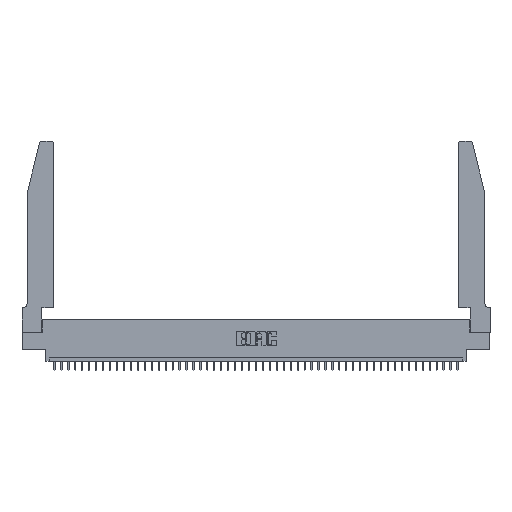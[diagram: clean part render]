
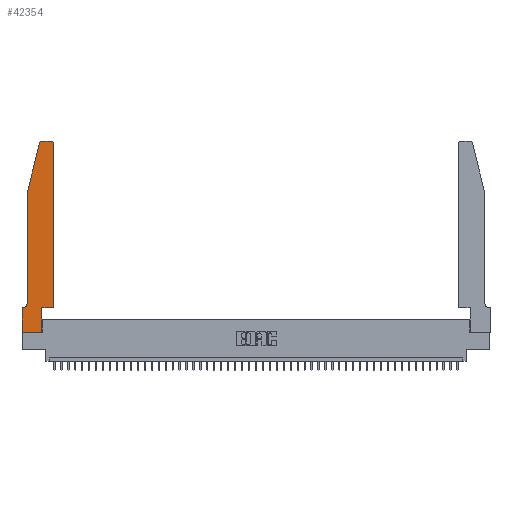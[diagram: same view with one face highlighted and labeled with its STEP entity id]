
A CAD part, top view. The second image highlights one B-rep face of the part: STEP entity #42354.
In plain terms, the highlighted planar face has unit normal (0, 0, 1).
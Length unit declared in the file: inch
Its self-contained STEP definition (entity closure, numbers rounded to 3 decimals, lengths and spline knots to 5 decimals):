
#681 = ORIENTED_EDGE ( 'NONE', *, *, #24891, .T. ) ;
#695 = CARTESIAN_POINT ( 'NONE',  ( 0.2865, 0., 0.37 ) ) ;
#1865 = CARTESIAN_POINT ( 'NONE',  ( 0.2865, 0.35, 0.37 ) ) ;
#1899 = EDGE_CURVE ( 'NONE', #6801, #45383, #42793, .T. ) ;
#1970 = DIRECTION ( 'NONE',  ( 0., 1., 0. ) ) ;
#2042 = EDGE_CURVE ( 'NONE', #19878, #34717, #4659, .T. ) ;
#2085 = VECTOR ( 'NONE', #27635, 39.37008 ) ;
#2311 = EDGE_CURVE ( 'NONE', #34717, #32950, #13893, .T. ) ;
#2432 = CARTESIAN_POINT ( 'NONE',  ( 0.2865, 0.35, 0.37 ) ) ;
#2750 = EDGE_CURVE ( 'NONE', #32636, #19404, #9795, .T. ) ;
#2810 = ORIENTED_EDGE ( 'NONE', *, *, #10127, .T. ) ;
#3376 = ORIENTED_EDGE ( 'NONE', *, *, #11991, .T. ) ;
#3710 = CARTESIAN_POINT ( 'NONE',  ( 0.2605, 2.75, 0.37 ) ) ;
#4659 = LINE ( 'NONE', #19162, #28533 ) ;
#5027 = AXIS2_PLACEMENT_3D ( 'NONE', #43188, #36262, #32211 ) ;
#6279 = DIRECTION ( 'NONE',  ( 0., 0., 1. ) ) ;
#6488 = DIRECTION ( 'NONE',  ( 1., 0., 0. ) ) ;
#6801 = VERTEX_POINT ( 'NONE', #29348 ) ;
#7514 = CARTESIAN_POINT ( 'NONE',  ( 0.4505, 2.72, 0.37 ) ) ;
#7860 = LINE ( 'NONE', #22376, #17465 ) ;
#8161 = DIRECTION ( 'NONE',  ( 1., 0., 0. ) ) ;
#8250 = ORIENTED_EDGE ( 'NONE', *, *, #2042, .T. ) ;
#8858 = CIRCLE ( 'NONE', #11123, 0.07 ) ;
#8876 = LINE ( 'NONE', #44636, #16606 ) ;
#9313 = LINE ( 'NONE', #38373, #2085 ) ;
#9795 = LINE ( 'NONE', #31712, #18900 ) ;
#9813 = LINE ( 'NONE', #2432, #31734 ) ;
#9866 = VECTOR ( 'NONE', #10618, 39.37008 ) ;
#10078 = CARTESIAN_POINT ( 'NONE',  ( 0., 0., 0.37 ) ) ;
#10095 = ORIENTED_EDGE ( 'NONE', *, *, #46100, .T. ) ;
#10127 = EDGE_CURVE ( 'NONE', #16687, #29132, #9813, .T. ) ;
#10618 = DIRECTION ( 'NONE',  ( -1., 0., 0. ) ) ;
#11123 = AXIS2_PLACEMENT_3D ( 'NONE', #24997, #31701, #39310 ) ;
#11627 = ORIENTED_EDGE ( 'NONE', *, *, #2750, .T. ) ;
#11991 = EDGE_CURVE ( 'NONE', #43808, #40932, #9313, .T. ) ;
#13331 = CARTESIAN_POINT ( 'NONE',  ( 0.0055, 0.35, 0.37 ) ) ;
#13660 = CARTESIAN_POINT ( 'NONE',  ( 0., 0., 0.37 ) ) ;
#13893 = LINE ( 'NONE', #13660, #29370 ) ;
#14557 = EDGE_CURVE ( 'NONE', #29132, #43808, #7860, .T. ) ;
#16606 = VECTOR ( 'NONE', #8161, 39.37008 ) ;
#16687 = VERTEX_POINT ( 'NONE', #695 ) ;
#16917 = ORIENTED_EDGE ( 'NONE', *, *, #1899, .T. ) ;
#17465 = VECTOR ( 'NONE', #6488, 39.37008 ) ;
#17757 = CARTESIAN_POINT ( 'NONE',  ( 0., 0.35, 0.37 ) ) ;
#18342 = CARTESIAN_POINT ( 'NONE',  ( 0., 0.35, 0.37 ) ) ;
#18900 = VECTOR ( 'NONE', #20962, 39.37008 ) ;
#19162 = CARTESIAN_POINT ( 'NONE',  ( 0.0755, 0.35, 0.37 ) ) ;
#19404 = VERTEX_POINT ( 'NONE', #20272 ) ;
#19878 = VERTEX_POINT ( 'NONE', #13331 ) ;
#20091 = CARTESIAN_POINT ( 'NONE',  ( 0.4205, 2.72, 0.37 ) ) ;
#20272 = CARTESIAN_POINT ( 'NONE',  ( 0.0755, 2., 0.37 ) ) ;
#20962 = DIRECTION ( 'NONE',  ( -0.239, -0.971, 0. ) ) ;
#21326 = FACE_OUTER_BOUND ( 'NONE', #31889, .T. ) ;
#21738 = ORIENTED_EDGE ( 'NONE', *, *, #45630, .T. ) ;
#22376 = CARTESIAN_POINT ( 'NONE',  ( 0.4505, 0.35, 0.37 ) ) ;
#23330 = CARTESIAN_POINT ( 'NONE',  ( 0.0755, 0.42, 0.37 ) ) ;
#23818 = VECTOR ( 'NONE', #33540, 39.37008 ) ;
#24444 = VERTEX_POINT ( 'NONE', #23330 ) ;
#24891 = EDGE_CURVE ( 'NONE', #40932, #6801, #43857, .T. ) ;
#24997 = CARTESIAN_POINT ( 'NONE',  ( 0.0055, 0.42, 0.37 ) ) ;
#27635 = DIRECTION ( 'NONE',  ( 0., 1., 0. ) ) ;
#28533 = VECTOR ( 'NONE', #36586, 39.37008 ) ;
#28964 = DIRECTION ( 'NONE',  ( 1., 0., 0. ) ) ;
#29119 = AXIS2_PLACEMENT_3D ( 'NONE', #17757, #32294, #28964 ) ;
#29132 = VERTEX_POINT ( 'NONE', #1865 ) ;
#29185 = CARTESIAN_POINT ( 'NONE',  ( 0.25487, 2.72718, 0.37 ) ) ;
#29348 = CARTESIAN_POINT ( 'NONE',  ( 0.4205, 2.75, 0.37 ) ) ;
#29370 = VECTOR ( 'NONE', #42504, 39.37008 ) ;
#29670 = ORIENTED_EDGE ( 'NONE', *, *, #42015, .T. ) ;
#30449 = CARTESIAN_POINT ( 'NONE',  ( 0.0755, 2., 0.37 ) ) ;
#30914 = LINE ( 'NONE', #30449, #23818 ) ;
#31292 = DIRECTION ( 'NONE',  ( 1., 0., 0. ) ) ;
#31537 = ORIENTED_EDGE ( 'NONE', *, *, #35622, .T. ) ;
#31701 = DIRECTION ( 'NONE',  ( 0., 0., -1. ) ) ;
#31712 = CARTESIAN_POINT ( 'NONE',  ( 0.0755, 2., 0.37 ) ) ;
#31734 = VECTOR ( 'NONE', #1970, 39.37008 ) ;
#31889 = EDGE_LOOP ( 'NONE', ( #16917, #21738, #11627, #29670, #10095, #8250, #38576, #31537, #2810, #39678, #3376, #681 ) ) ;
#32211 = DIRECTION ( 'NONE',  ( 1., 0., 0. ) ) ;
#32294 = DIRECTION ( 'NONE',  ( 0., 0., 1. ) ) ;
#32636 = VERTEX_POINT ( 'NONE', #29185 ) ;
#32950 = VERTEX_POINT ( 'NONE', #10078 ) ;
#33540 = DIRECTION ( 'NONE',  ( 0., -1., 0. ) ) ;
#33746 = CARTESIAN_POINT ( 'NONE',  ( 0.4505, 0.35, 0.37 ) ) ;
#34717 = VERTEX_POINT ( 'NONE', #18342 ) ;
#35622 = EDGE_CURVE ( 'NONE', #32950, #16687, #8876, .T. ) ;
#35871 = PLANE ( 'NONE',  #29119 ) ;
#36262 = DIRECTION ( 'NONE',  ( 0., 0., 1. ) ) ;
#36586 = DIRECTION ( 'NONE',  ( -1., 0., 0. ) ) ;
#38373 = CARTESIAN_POINT ( 'NONE',  ( 0.4505, 0.35, 0.37 ) ) ;
#38576 = ORIENTED_EDGE ( 'NONE', *, *, #2311, .T. ) ;
#39310 = DIRECTION ( 'NONE',  ( -1., 0., 0. ) ) ;
#39678 = ORIENTED_EDGE ( 'NONE', *, *, #14557, .T. ) ;
#40746 = CIRCLE ( 'NONE', #5027, 0.03 ) ;
#40932 = VERTEX_POINT ( 'NONE', #7514 ) ;
#41575 = AXIS2_PLACEMENT_3D ( 'NONE', #20091, #6279, #31292 ) ;
#42015 = EDGE_CURVE ( 'NONE', #19404, #24444, #30914, .T. ) ;
#42354 = ADVANCED_FACE ( 'NONE', ( #21326 ), #35871, .T. ) ;
#42504 = DIRECTION ( 'NONE',  ( 0., -1., 0. ) ) ;
#42793 = LINE ( 'NONE', #3710, #9866 ) ;
#43188 = CARTESIAN_POINT ( 'NONE',  ( 0.284, 2.72, 0.37 ) ) ;
#43808 = VERTEX_POINT ( 'NONE', #33746 ) ;
#43857 = CIRCLE ( 'NONE', #41575, 0.03 ) ;
#44205 = CARTESIAN_POINT ( 'NONE',  ( 0.284, 2.75, 0.37 ) ) ;
#44636 = CARTESIAN_POINT ( 'NONE',  ( 0., 0., 0.37 ) ) ;
#45383 = VERTEX_POINT ( 'NONE', #44205 ) ;
#45630 = EDGE_CURVE ( 'NONE', #45383, #32636, #40746, .T. ) ;
#46100 = EDGE_CURVE ( 'NONE', #24444, #19878, #8858, .T. ) ;
